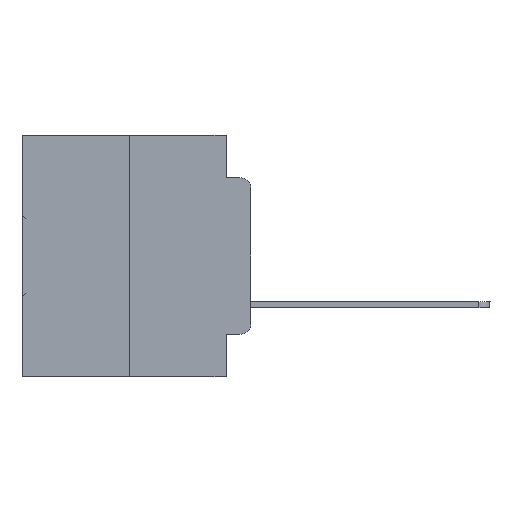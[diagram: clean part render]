
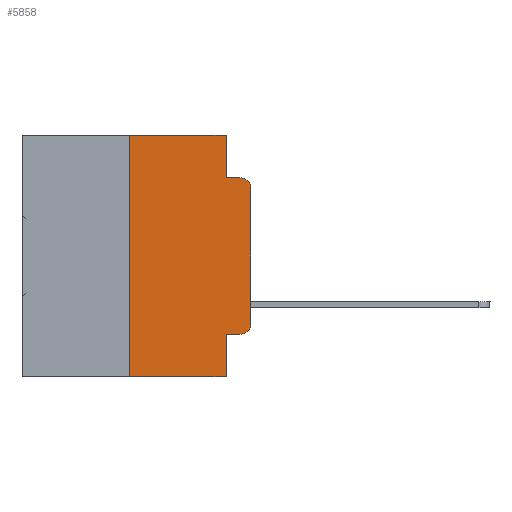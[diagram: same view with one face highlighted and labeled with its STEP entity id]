
A CAD part, left-side view. The second image highlights one B-rep face of the part: STEP entity #5858.
In plain terms, the highlighted planar face has unit normal (-1, 0, 0).
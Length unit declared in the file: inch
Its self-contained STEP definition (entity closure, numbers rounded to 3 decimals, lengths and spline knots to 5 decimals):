
#829 = DIRECTION ( 'NONE',  ( 0., 0., -1. ) ) ;
#1742 = VECTOR ( 'NONE', #9204, 39.37008 ) ;
#1791 = EDGE_CURVE ( 'NONE', #2764, #14250, #10128, .T. ) ;
#2307 = EDGE_CURVE ( 'NONE', #9397, #5277, #8868, .T. ) ;
#2764 = VERTEX_POINT ( 'NONE', #4945 ) ;
#2837 = CARTESIAN_POINT ( 'NONE',  ( 0., 0.051, -0.5 ) ) ;
#3648 = VERTEX_POINT ( 'NONE', #13513 ) ;
#4086 = ORIENTED_EDGE ( 'NONE', *, *, #2307, .F. ) ;
#4598 = VECTOR ( 'NONE', #10194, 39.37008 ) ;
#4945 = CARTESIAN_POINT ( 'NONE',  ( 0., 0., -0.3915 ) ) ;
#5277 = VERTEX_POINT ( 'NONE', #12923 ) ;
#5424 = ORIENTED_EDGE ( 'NONE', *, *, #31231, .T. ) ;
#5607 = LINE ( 'NONE', #30114, #18788 ) ;
#5858 = ADVANCED_FACE ( 'NONE', ( #17323 ), #28324, .F. ) ;
#6336 = VERTEX_POINT ( 'NONE', #9720 ) ;
#6567 = DIRECTION ( 'NONE',  ( 0., -1., 0. ) ) ;
#7226 = AXIS2_PLACEMENT_3D ( 'NONE', #13954, #29657, #32466 ) ;
#7607 = LINE ( 'NONE', #22964, #24536 ) ;
#8629 = DIRECTION ( 'NONE',  ( 0., 0., 1. ) ) ;
#8868 = LINE ( 'NONE', #29110, #10921 ) ;
#9204 = DIRECTION ( 'NONE',  ( 0., -1., 0. ) ) ;
#9397 = VERTEX_POINT ( 'NONE', #22524 ) ;
#9720 = CARTESIAN_POINT ( 'NONE',  ( 0., 0.02, -0.4115 ) ) ;
#9841 = EDGE_CURVE ( 'NONE', #14293, #26951, #26053, .T. ) ;
#10128 = LINE ( 'NONE', #20977, #20056 ) ;
#10179 = VECTOR ( 'NONE', #8629, 39.37008 ) ;
#10194 = DIRECTION ( 'NONE',  ( 0., -1., 0. ) ) ;
#10426 = CARTESIAN_POINT ( 'NONE',  ( 0., 0.25, 0. ) ) ;
#10449 = DIRECTION ( 'NONE',  ( 0., 0., 1. ) ) ;
#10921 = VECTOR ( 'NONE', #29230, 39.37008 ) ;
#11179 = CARTESIAN_POINT ( 'NONE',  ( 0., 0.25, 0. ) ) ;
#11566 = CIRCLE ( 'NONE', #12384, 0.02 ) ;
#12380 = EDGE_CURVE ( 'NONE', #14293, #24703, #30041, .T. ) ;
#12384 = AXIS2_PLACEMENT_3D ( 'NONE', #27125, #13747, #829 ) ;
#12781 = DIRECTION ( 'NONE',  ( 0., -1., 0. ) ) ;
#12923 = CARTESIAN_POINT ( 'NONE',  ( 0., 0.051, -0.0885 ) ) ;
#12994 = CARTESIAN_POINT ( 'NONE',  ( 0., 0.473, 0. ) ) ;
#13228 = CARTESIAN_POINT ( 'NONE',  ( 0., 0., -0.1085 ) ) ;
#13513 = CARTESIAN_POINT ( 'NONE',  ( 0., 0.02, -0.0885 ) ) ;
#13747 = DIRECTION ( 'NONE',  ( -1., 0., 0. ) ) ;
#13954 = CARTESIAN_POINT ( 'NONE',  ( 0., 0.02, -0.3915 ) ) ;
#14250 = VERTEX_POINT ( 'NONE', #13228 ) ;
#14293 = VERTEX_POINT ( 'NONE', #15984 ) ;
#15611 = ORIENTED_EDGE ( 'NONE', *, *, #17692, .T. ) ;
#15955 = LINE ( 'NONE', #33794, #27108 ) ;
#15984 = CARTESIAN_POINT ( 'NONE',  ( 0., 0.25, -0.5 ) ) ;
#16383 = ORIENTED_EDGE ( 'NONE', *, *, #1791, .T. ) ;
#16721 = ORIENTED_EDGE ( 'NONE', *, *, #9841, .T. ) ;
#17323 = FACE_OUTER_BOUND ( 'NONE', #24796, .T. ) ;
#17362 = CARTESIAN_POINT ( 'NONE',  ( 0., 0.051, -0.4115 ) ) ;
#17692 = EDGE_CURVE ( 'NONE', #14250, #3648, #11566, .T. ) ;
#18788 = VECTOR ( 'NONE', #6567, 39.37008 ) ;
#19682 = AXIS2_PLACEMENT_3D ( 'NONE', #12994, #28672, #26036 ) ;
#19829 = EDGE_CURVE ( 'NONE', #30182, #26951, #15955, .T. ) ;
#20056 = VECTOR ( 'NONE', #10449, 39.37008 ) ;
#20065 = CARTESIAN_POINT ( 'NONE',  ( 0., 0.051, -0.0885 ) ) ;
#20977 = CARTESIAN_POINT ( 'NONE',  ( 0., 0., 0. ) ) ;
#22524 = CARTESIAN_POINT ( 'NONE',  ( 0., 0.051, 0. ) ) ;
#22964 = CARTESIAN_POINT ( 'NONE',  ( 0., 0.473, 0. ) ) ;
#23853 = CARTESIAN_POINT ( 'NONE',  ( 0., 0.473, -0.5 ) ) ;
#24089 = EDGE_CURVE ( 'NONE', #24703, #9397, #7607, .T. ) ;
#24536 = VECTOR ( 'NONE', #12781, 39.37008 ) ;
#24703 = VERTEX_POINT ( 'NONE', #10426 ) ;
#24796 = EDGE_LOOP ( 'NONE', ( #16383, #15611, #31470, #4086, #32601, #30931, #16721, #30831, #33153, #5424 ) ) ;
#25566 = EDGE_CURVE ( 'NONE', #5277, #3648, #33998, .T. ) ;
#26036 = DIRECTION ( 'NONE',  ( 0., 0., -1. ) ) ;
#26053 = LINE ( 'NONE', #23853, #4598 ) ;
#26951 = VERTEX_POINT ( 'NONE', #2837 ) ;
#27108 = VECTOR ( 'NONE', #28759, 39.37008 ) ;
#27125 = CARTESIAN_POINT ( 'NONE',  ( 0., 0.02, -0.1085 ) ) ;
#27598 = CIRCLE ( 'NONE', #7226, 0.02 ) ;
#28324 = PLANE ( 'NONE',  #19682 ) ;
#28672 = DIRECTION ( 'NONE',  ( 1., 0., 0. ) ) ;
#28759 = DIRECTION ( 'NONE',  ( 0., 0., -1. ) ) ;
#29110 = CARTESIAN_POINT ( 'NONE',  ( 0., 0.051, 0. ) ) ;
#29230 = DIRECTION ( 'NONE',  ( 0., 0., -1. ) ) ;
#29657 = DIRECTION ( 'NONE',  ( -1., 0., 0. ) ) ;
#30041 = LINE ( 'NONE', #11179, #10179 ) ;
#30114 = CARTESIAN_POINT ( 'NONE',  ( 0., 0.051, -0.4115 ) ) ;
#30182 = VERTEX_POINT ( 'NONE', #17362 ) ;
#30831 = ORIENTED_EDGE ( 'NONE', *, *, #19829, .F. ) ;
#30931 = ORIENTED_EDGE ( 'NONE', *, *, #12380, .F. ) ;
#31231 = EDGE_CURVE ( 'NONE', #6336, #2764, #27598, .T. ) ;
#31470 = ORIENTED_EDGE ( 'NONE', *, *, #25566, .F. ) ;
#32466 = DIRECTION ( 'NONE',  ( 0., 0., -1. ) ) ;
#32601 = ORIENTED_EDGE ( 'NONE', *, *, #24089, .F. ) ;
#33153 = ORIENTED_EDGE ( 'NONE', *, *, #33419, .T. ) ;
#33419 = EDGE_CURVE ( 'NONE', #30182, #6336, #5607, .T. ) ;
#33794 = CARTESIAN_POINT ( 'NONE',  ( 0., 0.051, 0. ) ) ;
#33998 = LINE ( 'NONE', #20065, #1742 ) ;
